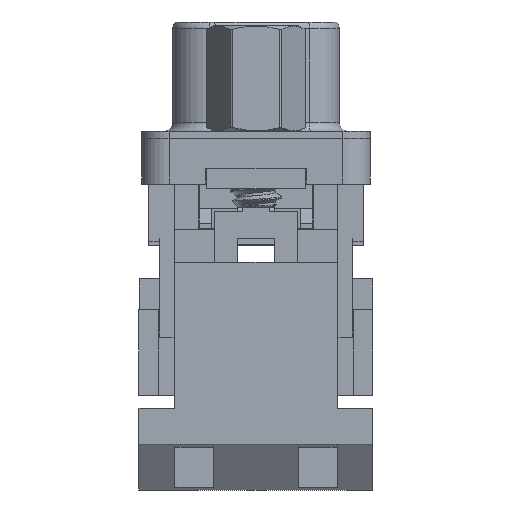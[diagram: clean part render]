
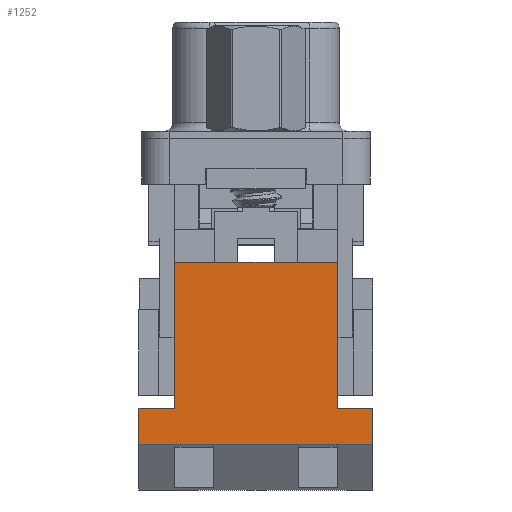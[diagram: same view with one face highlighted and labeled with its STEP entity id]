
A CAD part, left-side view. The second image highlights one B-rep face of the part: STEP entity #1252.
In plain terms, the highlighted planar face has unit normal (-1, 0, 0).
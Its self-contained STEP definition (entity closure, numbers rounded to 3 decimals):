
#14 = EDGE_CURVE ( 'NONE', #10250, #38845, #21869, .T. ) ;
#19 = LINE ( 'NONE', #468, #14055 ) ;
#342 = CARTESIAN_POINT ( 'NONE',  ( 3.245, -4.45, -6.8 ) ) ;
#468 = CARTESIAN_POINT ( 'NONE',  ( 3.245, 4.45, -6.8 ) ) ;
#1252 = ADVANCED_FACE ( 'NONE', ( #7566 ), #40420, .F. ) ;
#1321 = CARTESIAN_POINT ( 'NONE',  ( 3.245, -6.425, -15.3 ) ) ;
#1793 = CARTESIAN_POINT ( 'NONE',  ( 3.245, -4.45, -6.8 ) ) ;
#2423 = LINE ( 'NONE', #42164, #19288 ) ;
#2689 = EDGE_CURVE ( 'NONE', #10250, #40389, #2423, .T. ) ;
#2893 = VERTEX_POINT ( 'NONE', #33716 ) ;
#3179 = VECTOR ( 'NONE', #14640, 1000. ) ;
#3180 = CARTESIAN_POINT ( 'NONE',  ( 3.245, 4.45, -6.8 ) ) ;
#3569 = DIRECTION ( 'NONE',  ( 0., 0., -1. ) ) ;
#3787 = ORIENTED_EDGE ( 'NONE', *, *, #14535, .T. ) ;
#6931 = LINE ( 'NONE', #26024, #31589 ) ;
#7566 = FACE_OUTER_BOUND ( 'NONE', #13717, .T. ) ;
#8393 = CARTESIAN_POINT ( 'NONE',  ( 3.245, 6.425, -15.3 ) ) ;
#9387 = VERTEX_POINT ( 'NONE', #12886 ) ;
#9962 = DIRECTION ( 'NONE',  ( 0., 0., -1. ) ) ;
#10250 = VERTEX_POINT ( 'NONE', #23602 ) ;
#10447 = CARTESIAN_POINT ( 'NONE',  ( 3.245, 6.425, -14.8 ) ) ;
#11318 = ORIENTED_EDGE ( 'NONE', *, *, #11390, .F. ) ;
#11390 = EDGE_CURVE ( 'NONE', #22608, #9387, #33197, .T. ) ;
#12886 = CARTESIAN_POINT ( 'NONE',  ( 3.245, -4.45, -14.8 ) ) ;
#13059 = LINE ( 'NONE', #3180, #33003 ) ;
#13717 = EDGE_LOOP ( 'NONE', ( #17592, #22212, #27380, #26745, #11318, #40693, #3787, #29562 ) ) ;
#14055 = VECTOR ( 'NONE', #24287, 1000. ) ;
#14535 = EDGE_CURVE ( 'NONE', #2893, #40389, #13059, .T. ) ;
#14640 = DIRECTION ( 'NONE',  ( 0., 0., -1. ) ) ;
#15943 = VECTOR ( 'NONE', #37181, 1000. ) ;
#16962 = CARTESIAN_POINT ( 'NONE',  ( 3.245, -6.425, -16.8 ) ) ;
#17085 = DIRECTION ( 'NONE',  ( 0., -1., 0. ) ) ;
#17592 = ORIENTED_EDGE ( 'NONE', *, *, #14, .T. ) ;
#19020 = VECTOR ( 'NONE', #3569, 1000. ) ;
#19288 = VECTOR ( 'NONE', #31631, 1000. ) ;
#21869 = LINE ( 'NONE', #8393, #3179 ) ;
#22212 = ORIENTED_EDGE ( 'NONE', *, *, #31832, .F. ) ;
#22608 = VERTEX_POINT ( 'NONE', #1793 ) ;
#22936 = DIRECTION ( 'NONE',  ( 0., 0., -1. ) ) ;
#23602 = CARTESIAN_POINT ( 'NONE',  ( 3.245, 6.425, -14.8 ) ) ;
#23697 = VERTEX_POINT ( 'NONE', #40078 ) ;
#24287 = DIRECTION ( 'NONE',  ( 0., -1., 0. ) ) ;
#25134 = VERTEX_POINT ( 'NONE', #16962 ) ;
#26024 = CARTESIAN_POINT ( 'NONE',  ( 3.245, -6.425, -15.3 ) ) ;
#26745 = ORIENTED_EDGE ( 'NONE', *, *, #27752, .F. ) ;
#27038 = CARTESIAN_POINT ( 'NONE',  ( 3.245, 4.45, -14.8 ) ) ;
#27380 = ORIENTED_EDGE ( 'NONE', *, *, #28088, .F. ) ;
#27752 = EDGE_CURVE ( 'NONE', #9387, #23697, #39859, .T. ) ;
#28088 = EDGE_CURVE ( 'NONE', #23697, #25134, #6931, .T. ) ;
#29562 = ORIENTED_EDGE ( 'NONE', *, *, #2689, .F. ) ;
#30201 = VECTOR ( 'NONE', #17085, 1000. ) ;
#31589 = VECTOR ( 'NONE', #9962, 1000. ) ;
#31631 = DIRECTION ( 'NONE',  ( 0., -1., 0. ) ) ;
#31832 = EDGE_CURVE ( 'NONE', #25134, #38845, #34356, .T. ) ;
#33003 = VECTOR ( 'NONE', #22936, 1000. ) ;
#33197 = LINE ( 'NONE', #342, #19020 ) ;
#33716 = CARTESIAN_POINT ( 'NONE',  ( 3.245, 4.45, -6.8 ) ) ;
#34356 = LINE ( 'NONE', #40833, #15943 ) ;
#35319 = CARTESIAN_POINT ( 'NONE',  ( 3.245, 6.425, -16.8 ) ) ;
#36775 = DIRECTION ( 'NONE',  ( 1., 0., 0. ) ) ;
#37181 = DIRECTION ( 'NONE',  ( 0., 1., 0. ) ) ;
#37405 = DIRECTION ( 'NONE',  ( 0., 0., -1. ) ) ;
#38214 = EDGE_CURVE ( 'NONE', #2893, #22608, #19, .T. ) ;
#38702 = AXIS2_PLACEMENT_3D ( 'NONE', #1321, #36775, #37405 ) ;
#38845 = VERTEX_POINT ( 'NONE', #35319 ) ;
#39859 = LINE ( 'NONE', #10447, #30201 ) ;
#40078 = CARTESIAN_POINT ( 'NONE',  ( 3.245, -6.425, -14.8 ) ) ;
#40389 = VERTEX_POINT ( 'NONE', #27038 ) ;
#40420 = PLANE ( 'NONE',  #38702 ) ;
#40693 = ORIENTED_EDGE ( 'NONE', *, *, #38214, .F. ) ;
#40833 = CARTESIAN_POINT ( 'NONE',  ( 3.245, -6.425, -16.8 ) ) ;
#42164 = CARTESIAN_POINT ( 'NONE',  ( 3.245, 6.425, -14.8 ) ) ;
